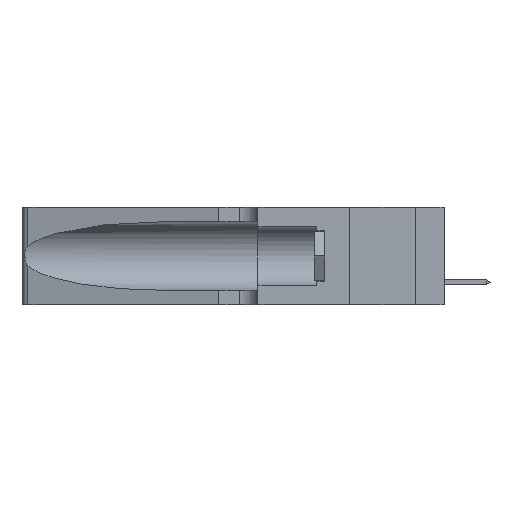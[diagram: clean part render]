
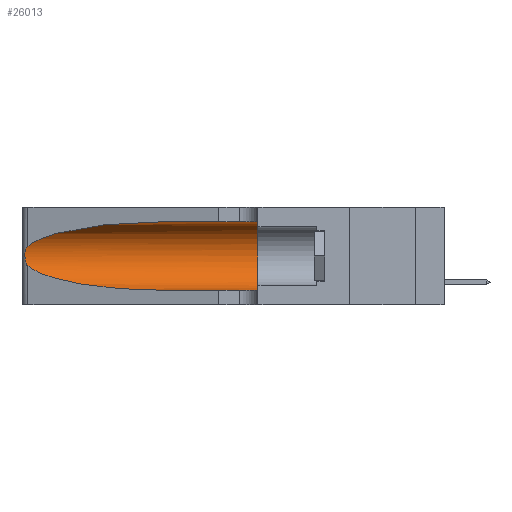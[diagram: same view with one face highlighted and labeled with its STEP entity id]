
A CAD part, left-side view. The second image highlights one B-rep face of the part: STEP entity #26013.
In plain terms, the highlighted cylindrical face has radius 3.308 mm (diameter 6.617 mm), a partial arc.
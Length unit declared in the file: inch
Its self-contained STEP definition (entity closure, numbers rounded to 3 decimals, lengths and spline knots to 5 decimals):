
#222 = EDGE_CURVE ( 'NONE', #16201, #21044, #35866, .T. ) ;
#1838 = DIRECTION ( 'NONE',  ( 0., -1., 0. ) ) ;
#1839 = DIRECTION ( 'NONE',  ( 0., -1., 0. ) ) ;
#3258 = CARTESIAN_POINT ( 'NONE',  ( 0.25487, 1.22718, 0.14631 ) ) ;
#3730 =( BOUNDED_CURVE ( )  B_SPLINE_CURVE ( 3, ( #29533, #23812, #6494, #23681 ),
 .UNSPECIFIED., .F., .F. ) 
 B_SPLINE_CURVE_WITH_KNOTS ( ( 4, 4 ),
 ( 3.44316, 4.71239 ),
 .UNSPECIFIED. ) 
 CURVE ( )  GEOMETRIC_REPRESENTATION_ITEM ( )  RATIONAL_B_SPLINE_CURVE ( ( 1., 0.87, 0.87, 1. ) ) 
 REPRESENTATION_ITEM ( '' )  );
#4325 = EDGE_CURVE ( 'NONE', #16201, #32301, #5382, .T. ) ;
#4672 = AXIS2_PLACEMENT_3D ( 'NONE', #5255, #24726, #30827 ) ;
#4823 = CARTESIAN_POINT ( 'NONE',  ( 0.25789, 1.23486, 0.15765 ) ) ;
#4863 = CARTESIAN_POINT ( 'NONE',  ( 0.1305, 1.61858, 0.185 ) ) ;
#4922 = CARTESIAN_POINT ( 'NONE',  ( 0.1305, 0.72297, 0.31525 ) ) ;
#5209 = CARTESIAN_POINT ( 'NONE',  ( 0.26075, 1.23896, 0.178 ) ) ;
#5223 = EDGE_CURVE ( 'NONE', #26456, #25176, #30136, .T. ) ;
#5255 = CARTESIAN_POINT ( 'NONE',  ( 0.1305, 0.35, 0.185 ) ) ;
#5382 =( BOUNDED_CURVE ( )  B_SPLINE_CURVE ( 3, ( #20772, #17667, #34645, #36122 ),
 .UNSPECIFIED., .F., .F. ) 
 B_SPLINE_CURVE_WITH_KNOTS ( ( 4, 4 ),
 ( 1.5708, 2.84003 ),
 .UNSPECIFIED. ) 
 CURVE ( )  GEOMETRIC_REPRESENTATION_ITEM ( )  RATIONAL_B_SPLINE_CURVE ( ( 1., 0.87, 0.87, 1. ) ) 
 REPRESENTATION_ITEM ( '' )  );
#5767 = EDGE_LOOP ( 'NONE', ( #18443, #28464, #9217, #31397, #28766, #25733 ) ) ;
#5887 = AXIS2_PLACEMENT_3D ( 'NONE', #4863, #1838, #19380 ) ;
#6494 = CARTESIAN_POINT ( 'NONE',  ( 0.18966, 0.96281, 0.05475 ) ) ;
#7014 = CARTESIAN_POINT ( 'NONE',  ( 0.1305, 1.61858, 0.05475 ) ) ;
#7717 = CARTESIAN_POINT ( 'NONE',  ( 0.26018, 1.23835, 0.19895 ) ) ;
#7849 = CARTESIAN_POINT ( 'NONE',  ( 0.26017, 1.23833, 0.17102 ) ) ;
#7901 = CARTESIAN_POINT ( 'NONE',  ( 0.1305, 1.61858, 0.31525 ) ) ;
#7975 = CARTESIAN_POINT ( 'NONE',  ( 0.25555, 1.22994, 0.2215 ) ) ;
#8227 = CARTESIAN_POINT ( 'NONE',  ( 0.25787, 1.23484, 0.2124 ) ) ;
#9217 = ORIENTED_EDGE ( 'NONE', *, *, #9643, .T. ) ;
#9643 = EDGE_CURVE ( 'NONE', #32601, #26456, #3730, .T. ) ;
#9955 = CYLINDRICAL_SURFACE ( 'NONE', #5887, 0.13025 ) ;
#10826 = FACE_OUTER_BOUND ( 'NONE', #5767, .T. ) ;
#11264 = CIRCLE ( 'NONE', #4672, 0.13025 ) ;
#13823 = CARTESIAN_POINT ( 'NONE',  ( 0.25856, 1.23593, 0.16098 ) ) ;
#13954 = VECTOR ( 'NONE', #1839, 39.37008 ) ;
#15599 = CARTESIAN_POINT ( 'NONE',  ( 0.1305, 0.35, 0.05475 ) ) ;
#16201 = VERTEX_POINT ( 'NONE', #4922 ) ;
#16585 = CARTESIAN_POINT ( 'NONE',  ( 0.25639, 1.23184, 0.21858 ) ) ;
#17667 = CARTESIAN_POINT ( 'NONE',  ( 0.18966, 0.96281, 0.31525 ) ) ;
#18443 = ORIENTED_EDGE ( 'NONE', *, *, #4325, .T. ) ;
#19169 = CARTESIAN_POINT ( 'NONE',  ( 0.25487, 1.22718, 0.22369 ) ) ;
#19330 = CARTESIAN_POINT ( 'NONE',  ( 0.25487, 1.22718, 0.22369 ) ) ;
#19380 = DIRECTION ( 'NONE',  ( 0., 0., -1. ) ) ;
#19579 = CARTESIAN_POINT ( 'NONE',  ( 0.26075, 1.23896, 0.19203 ) ) ;
#20276 = CARTESIAN_POINT ( 'NONE',  ( 0.1305, 0.35, 0.31525 ) ) ;
#20772 = CARTESIAN_POINT ( 'NONE',  ( 0.1305, 0.72297, 0.31525 ) ) ;
#21044 = VERTEX_POINT ( 'NONE', #20276 ) ;
#21372 = DIRECTION ( 'NONE',  ( 0., -1., 0. ) ) ;
#22203 = CARTESIAN_POINT ( 'NONE',  ( 0.25487, 1.22718, 0.14631 ) ) ;
#23681 = CARTESIAN_POINT ( 'NONE',  ( 0.1305, 0.72297, 0.05475 ) ) ;
#23812 = CARTESIAN_POINT ( 'NONE',  ( 0.2373, 1.15595, 0.08982 ) ) ;
#24726 = DIRECTION ( 'NONE',  ( 0., 1., 0. ) ) ;
#25176 = VERTEX_POINT ( 'NONE', #15599 ) ;
#25733 = ORIENTED_EDGE ( 'NONE', *, *, #222, .F. ) ;
#25988 = EDGE_CURVE ( 'NONE', #21044, #25176, #11264, .T. ) ;
#26013 = ADVANCED_FACE ( 'NONE', ( #10826 ), #9955, .F. ) ;
#26456 = VERTEX_POINT ( 'NONE', #28047 ) ;
#28047 = CARTESIAN_POINT ( 'NONE',  ( 0.1305, 0.72297, 0.05475 ) ) ;
#28464 = ORIENTED_EDGE ( 'NONE', *, *, #36478, .T. ) ;
#28689 = B_SPLINE_CURVE_WITH_KNOTS ( 'NONE', 3,
 ( #19330, #7975, #16585, #8227, #30909, #7717, #19579, #5209, #7849, #13823, #4823, #36447, #30398, #22203 ),
 .UNSPECIFIED., .F., .F.,
 ( 4, 2, 2, 2, 2, 2, 4 ),
 ( 0., 0.00027, 0.00053, 0.00107, 0.0016, 0.00187, 0.00214 ),
 .UNSPECIFIED. ) ;
#28766 = ORIENTED_EDGE ( 'NONE', *, *, #25988, .F. ) ;
#29533 = CARTESIAN_POINT ( 'NONE',  ( 0.25487, 1.22718, 0.14631 ) ) ;
#30136 = LINE ( 'NONE', #7014, #35999 ) ;
#30398 = CARTESIAN_POINT ( 'NONE',  ( 0.25555, 1.22993, 0.14849 ) ) ;
#30827 = DIRECTION ( 'NONE',  ( 0., 0., 1. ) ) ;
#30909 = CARTESIAN_POINT ( 'NONE',  ( 0.25854, 1.2359, 0.20912 ) ) ;
#31397 = ORIENTED_EDGE ( 'NONE', *, *, #5223, .T. ) ;
#32301 = VERTEX_POINT ( 'NONE', #19169 ) ;
#32601 = VERTEX_POINT ( 'NONE', #3258 ) ;
#34645 = CARTESIAN_POINT ( 'NONE',  ( 0.2373, 1.15595, 0.28018 ) ) ;
#35866 = LINE ( 'NONE', #7901, #13954 ) ;
#35999 = VECTOR ( 'NONE', #21372, 39.37008 ) ;
#36122 = CARTESIAN_POINT ( 'NONE',  ( 0.25487, 1.22718, 0.22369 ) ) ;
#36447 = CARTESIAN_POINT ( 'NONE',  ( 0.25639, 1.23186, 0.15144 ) ) ;
#36478 = EDGE_CURVE ( 'NONE', #32301, #32601, #28689, .T. ) ;
